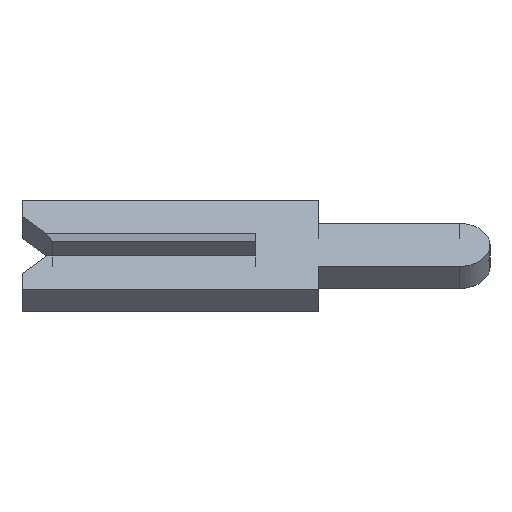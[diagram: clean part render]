
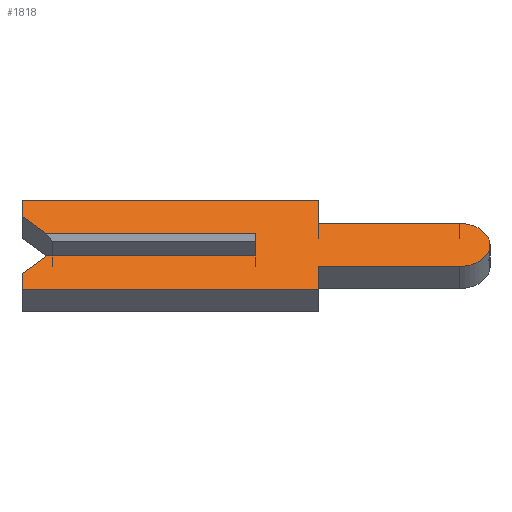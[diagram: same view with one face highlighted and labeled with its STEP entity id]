
A CAD part, left-side view. The second image highlights one B-rep face of the part: STEP entity #1818.
In plain terms, the highlighted face is planar.
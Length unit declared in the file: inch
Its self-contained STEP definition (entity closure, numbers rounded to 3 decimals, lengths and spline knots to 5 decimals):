
#22 = LINE ( 'NONE', #937, #1249 ) ;
#68 = DIRECTION ( 'NONE',  ( 0., -1., 0. ) ) ;
#74 = ORIENTED_EDGE ( 'NONE', *, *, #2155, .F. ) ;
#84 = LINE ( 'NONE', #177, #706 ) ;
#102 = CARTESIAN_POINT ( 'NONE',  ( -0.01, 0.15, 0.026 ) ) ;
#144 = EDGE_CURVE ( 'NONE', #313, #941, #1481, .T. ) ;
#161 = CARTESIAN_POINT ( 'NONE',  ( -0.01, -0.04, 0.0195 ) ) ;
#177 = CARTESIAN_POINT ( 'NONE',  ( -0.01, 0.15, 0.04 ) ) ;
#191 = AXIS2_PLACEMENT_3D ( 'NONE', #1482, #550, #2206 ) ;
#249 = EDGE_CURVE ( 'NONE', #2203, #1365, #546, .T. ) ;
#250 = CARTESIAN_POINT ( 'NONE',  ( -0.01, -0.04, -0.0195 ) ) ;
#290 = DIRECTION ( 'NONE',  ( 0., 0., 1. ) ) ;
#307 = EDGE_CURVE ( 'NONE', #1153, #1698, #1671, .T. ) ;
#313 = VERTEX_POINT ( 'NONE', #1183 ) ;
#333 = CARTESIAN_POINT ( 'NONE',  ( -0.01, 0.1305, 0.0065 ) ) ;
#341 = VECTOR ( 'NONE', #290, 39.37008 ) ;
#348 = ORIENTED_EDGE ( 'NONE', *, *, #1551, .F. ) ;
#371 = DIRECTION ( 'NONE',  ( 0., 0., 1. ) ) ;
#385 = EDGE_CURVE ( 'NONE', #1698, #1275, #1585, .T. ) ;
#389 = EDGE_LOOP ( 'NONE', ( #451, #2002, #2006, #2166, #1722, #888, #614, #1860, #74, #2104, #2291, #348, #524, #1252 ) ) ;
#396 = CARTESIAN_POINT ( 'NONE',  ( -0.01, 0.134, 0.01 ) ) ;
#446 = VERTEX_POINT ( 'NONE', #808 ) ;
#451 = ORIENTED_EDGE ( 'NONE', *, *, #249, .T. ) ;
#461 = VECTOR ( 'NONE', #1620, 39.37008 ) ;
#510 = EDGE_CURVE ( 'NONE', #856, #1157, #1532, .T. ) ;
#511 = CARTESIAN_POINT ( 'NONE',  ( -0.01, 0., -0.01 ) ) ;
#520 = CARTESIAN_POINT ( 'NONE',  ( -0.01, -0.04, -0.0195 ) ) ;
#524 = ORIENTED_EDGE ( 'NONE', *, *, #876, .F. ) ;
#546 = LINE ( 'NONE', #1901, #1309 ) ;
#550 = DIRECTION ( 'NONE',  ( 1., 0., 0. ) ) ;
#579 = CARTESIAN_POINT ( 'NONE',  ( -0.01, -0.1305, 0.0195 ) ) ;
#614 = ORIENTED_EDGE ( 'NONE', *, *, #385, .F. ) ;
#640 = CARTESIAN_POINT ( 'NONE',  ( -0.01, 0.15, -0.04 ) ) ;
#678 = CARTESIAN_POINT ( 'NONE',  ( -0.01, -0.04, 0.04 ) ) ;
#703 = CARTESIAN_POINT ( 'NONE',  ( -0.01, 0.15, -0.04 ) ) ;
#706 = VECTOR ( 'NONE', #1462, 39.37008 ) ;
#759 = CARTESIAN_POINT ( 'NONE',  ( -0.01, -0.1305, 0. ) ) ;
#762 = CIRCLE ( 'NONE', #924, 0.0195 ) ;
#788 = CARTESIAN_POINT ( 'NONE',  ( -0.01, -0.1305, -0.01 ) ) ;
#808 = CARTESIAN_POINT ( 'NONE',  ( -0.01, -0.04, 0.0195 ) ) ;
#811 = VERTEX_POINT ( 'NONE', #102 ) ;
#827 = CARTESIAN_POINT ( 'NONE',  ( -0.01, 0.15, -0.026 ) ) ;
#856 = VERTEX_POINT ( 'NONE', #640 ) ;
#876 = EDGE_CURVE ( 'NONE', #811, #2363, #1812, .T. ) ;
#888 = ORIENTED_EDGE ( 'NONE', *, *, #1724, .F. ) ;
#907 = DIRECTION ( 'NONE',  ( 0., 0., -1. ) ) ;
#924 = AXIS2_PLACEMENT_3D ( 'NONE', #759, #2260, #1339 ) ;
#937 = CARTESIAN_POINT ( 'NONE',  ( -0.01, 0.1305, -0.0065 ) ) ;
#941 = VERTEX_POINT ( 'NONE', #511 ) ;
#1002 = CARTESIAN_POINT ( 'NONE',  ( -0.01, 0.15, 0.04 ) ) ;
#1014 = DIRECTION ( 'NONE',  ( 0., 0., -1. ) ) ;
#1103 = VERTEX_POINT ( 'NONE', #678 ) ;
#1133 = LINE ( 'NONE', #333, #1709 ) ;
#1138 = CARTESIAN_POINT ( 'NONE',  ( -0.01, 0., 0.0065 ) ) ;
#1153 = VERTEX_POINT ( 'NONE', #2158 ) ;
#1157 = VERTEX_POINT ( 'NONE', #1788 ) ;
#1167 = CARTESIAN_POINT ( 'NONE',  ( -0.01, -0.04, -0.04 ) ) ;
#1183 = CARTESIAN_POINT ( 'NONE',  ( -0.01, 0.134, -0.01 ) ) ;
#1186 = LINE ( 'NONE', #1838, #1450 ) ;
#1217 = VECTOR ( 'NONE', #371, 39.37008 ) ;
#1249 = VECTOR ( 'NONE', #1694, 39.37008 ) ;
#1252 = ORIENTED_EDGE ( 'NONE', *, *, #1787, .F. ) ;
#1275 = VERTEX_POINT ( 'NONE', #1167 ) ;
#1305 = DIRECTION ( 'NONE',  ( 0., 1., 0. ) ) ;
#1306 = LINE ( 'NONE', #161, #1667 ) ;
#1309 = VECTOR ( 'NONE', #68, 39.37008 ) ;
#1339 = DIRECTION ( 'NONE',  ( 0., 0., -1. ) ) ;
#1365 = VERTEX_POINT ( 'NONE', #1379 ) ;
#1379 = CARTESIAN_POINT ( 'NONE',  ( -0.01, 0., 0.01 ) ) ;
#1450 = VECTOR ( 'NONE', #907, 39.37008 ) ;
#1462 = DIRECTION ( 'NONE',  ( 0., -1., 0. ) ) ;
#1481 = LINE ( 'NONE', #788, #1782 ) ;
#1482 = CARTESIAN_POINT ( 'NONE',  ( -0.01, -0.1305, 0. ) ) ;
#1516 = DIRECTION ( 'NONE',  ( 0., 1., 0. ) ) ;
#1532 = LINE ( 'NONE', #827, #341 ) ;
#1551 = EDGE_CURVE ( 'NONE', #2363, #1103, #84, .T. ) ;
#1585 = LINE ( 'NONE', #1725, #1957 ) ;
#1620 = DIRECTION ( 'NONE',  ( 0., 0., 1. ) ) ;
#1640 = DIRECTION ( 'NONE',  ( 0., -1., 0. ) ) ;
#1667 = VECTOR ( 'NONE', #1640, 39.37008 ) ;
#1671 = LINE ( 'NONE', #250, #2020 ) ;
#1694 = DIRECTION ( 'NONE',  ( 0., -0.707, 0.707 ) ) ;
#1695 = FACE_OUTER_BOUND ( 'NONE', #389, .T. ) ;
#1698 = VERTEX_POINT ( 'NONE', #520 ) ;
#1709 = VECTOR ( 'NONE', #2216, 39.37008 ) ;
#1722 = ORIENTED_EDGE ( 'NONE', *, *, #510, .F. ) ;
#1724 = EDGE_CURVE ( 'NONE', #1275, #856, #2202, .T. ) ;
#1725 = CARTESIAN_POINT ( 'NONE',  ( -0.01, -0.04, -0.04 ) ) ;
#1744 = EDGE_CURVE ( 'NONE', #1103, #446, #1186, .T. ) ;
#1782 = VECTOR ( 'NONE', #2073, 39.37008 ) ;
#1787 = EDGE_CURVE ( 'NONE', #2203, #811, #1133, .T. ) ;
#1788 = CARTESIAN_POINT ( 'NONE',  ( -0.01, 0.15, -0.026 ) ) ;
#1812 = LINE ( 'NONE', #1970, #461 ) ;
#1818 = ADVANCED_FACE ( 'NONE', ( #1695 ), #2194, .F. ) ;
#1838 = CARTESIAN_POINT ( 'NONE',  ( -0.01, -0.04, 0.04 ) ) ;
#1850 = EDGE_CURVE ( 'NONE', #941, #1365, #1868, .T. ) ;
#1860 = ORIENTED_EDGE ( 'NONE', *, *, #307, .F. ) ;
#1868 = LINE ( 'NONE', #1138, #1217 ) ;
#1870 = EDGE_CURVE ( 'NONE', #446, #1965, #1306, .T. ) ;
#1901 = CARTESIAN_POINT ( 'NONE',  ( -0.01, 0.15, 0.01 ) ) ;
#1957 = VECTOR ( 'NONE', #1014, 39.37008 ) ;
#1965 = VERTEX_POINT ( 'NONE', #579 ) ;
#1970 = CARTESIAN_POINT ( 'NONE',  ( -0.01, 0.15, 0.026 ) ) ;
#2002 = ORIENTED_EDGE ( 'NONE', *, *, #1850, .F. ) ;
#2006 = ORIENTED_EDGE ( 'NONE', *, *, #144, .F. ) ;
#2020 = VECTOR ( 'NONE', #1516, 39.37008 ) ;
#2073 = DIRECTION ( 'NONE',  ( 0., -1., 0. ) ) ;
#2104 = ORIENTED_EDGE ( 'NONE', *, *, #1870, .F. ) ;
#2137 = VECTOR ( 'NONE', #1305, 39.37008 ) ;
#2141 = EDGE_CURVE ( 'NONE', #1157, #313, #22, .T. ) ;
#2155 = EDGE_CURVE ( 'NONE', #1965, #1153, #762, .T. ) ;
#2158 = CARTESIAN_POINT ( 'NONE',  ( -0.01, -0.1305, -0.0195 ) ) ;
#2166 = ORIENTED_EDGE ( 'NONE', *, *, #2141, .F. ) ;
#2194 = PLANE ( 'NONE',  #191 ) ;
#2202 = LINE ( 'NONE', #703, #2137 ) ;
#2203 = VERTEX_POINT ( 'NONE', #396 ) ;
#2206 = DIRECTION ( 'NONE',  ( 0., 0., -1. ) ) ;
#2216 = DIRECTION ( 'NONE',  ( 0., 0.707, 0.707 ) ) ;
#2260 = DIRECTION ( 'NONE',  ( 1., 0., 0. ) ) ;
#2291 = ORIENTED_EDGE ( 'NONE', *, *, #1744, .F. ) ;
#2363 = VERTEX_POINT ( 'NONE', #1002 ) ;
